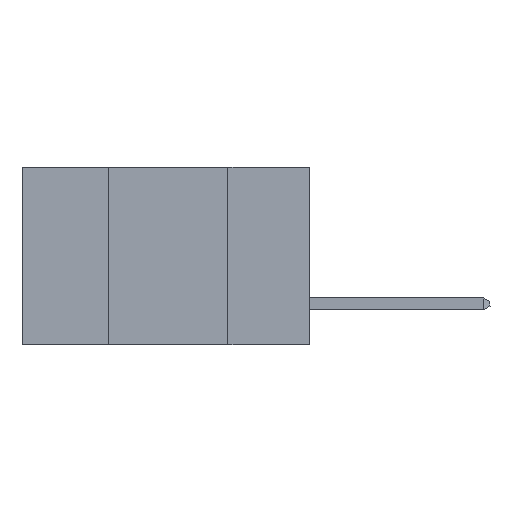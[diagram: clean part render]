
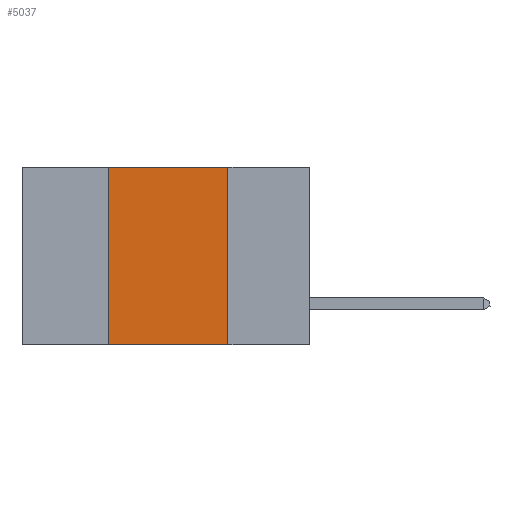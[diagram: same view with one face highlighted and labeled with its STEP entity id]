
A CAD part, left-side view. The second image highlights one B-rep face of the part: STEP entity #5037.
In plain terms, the highlighted planar face has unit normal (-1, 0, 0).
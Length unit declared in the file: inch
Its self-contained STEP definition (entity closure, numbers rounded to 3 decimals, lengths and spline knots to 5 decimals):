
#1005 = VECTOR ( 'NONE', #12761, 39.37008 ) ;
#1248 = FACE_OUTER_BOUND ( 'NONE', #7220, .T. ) ;
#1402 = LINE ( 'NONE', #6856, #10842 ) ;
#1527 = CARTESIAN_POINT ( 'NONE',  ( 0., 0.42, 0. ) ) ;
#2513 = LINE ( 'NONE', #8085, #5678 ) ;
#3950 = CARTESIAN_POINT ( 'NONE',  ( 0., 0.42, -0.37 ) ) ;
#4233 = LINE ( 'NONE', #4594, #1005 ) ;
#4409 = LINE ( 'NONE', #9572, #10308 ) ;
#4428 = VERTEX_POINT ( 'NONE', #9862 ) ;
#4594 = CARTESIAN_POINT ( 'NONE',  ( 0., 0.6, -0.37 ) ) ;
#4673 = AXIS2_PLACEMENT_3D ( 'NONE', #12328, #12309, #12293 ) ;
#4793 = ORIENTED_EDGE ( 'NONE', *, *, #11866, .F. ) ;
#5037 = ADVANCED_FACE ( 'NONE', ( #1248 ), #12649, .F. ) ;
#5542 = ORIENTED_EDGE ( 'NONE', *, *, #11166, .F. ) ;
#5675 = VERTEX_POINT ( 'NONE', #3950 ) ;
#5678 = VECTOR ( 'NONE', #8144, 39.37008 ) ;
#6143 = EDGE_CURVE ( 'NONE', #5675, #4428, #4233, .T. ) ;
#6856 = CARTESIAN_POINT ( 'NONE',  ( 0., 0.6, 0. ) ) ;
#7220 = EDGE_LOOP ( 'NONE', ( #4793, #5542, #12440, #10150 ) ) ;
#8085 = CARTESIAN_POINT ( 'NONE',  ( 0., 0.17, 0. ) ) ;
#8144 = DIRECTION ( 'NONE',  ( 0., 0., -1. ) ) ;
#8832 = VERTEX_POINT ( 'NONE', #1527 ) ;
#9268 = DIRECTION ( 'NONE',  ( 0., -1., 0. ) ) ;
#9572 = CARTESIAN_POINT ( 'NONE',  ( 0., 0.42, 0. ) ) ;
#9862 = CARTESIAN_POINT ( 'NONE',  ( 0., 0.17, -0.37 ) ) ;
#10150 = ORIENTED_EDGE ( 'NONE', *, *, #6143, .T. ) ;
#10308 = VECTOR ( 'NONE', #10802, 39.37008 ) ;
#10802 = DIRECTION ( 'NONE',  ( 0., 0., 1. ) ) ;
#10842 = VECTOR ( 'NONE', #9268, 39.37008 ) ;
#11166 = EDGE_CURVE ( 'NONE', #8832, #13412, #1402, .T. ) ;
#11349 = EDGE_CURVE ( 'NONE', #5675, #8832, #4409, .T. ) ;
#11866 = EDGE_CURVE ( 'NONE', #13412, #4428, #2513, .T. ) ;
#12293 = DIRECTION ( 'NONE',  ( 0., 0., -1. ) ) ;
#12309 = DIRECTION ( 'NONE',  ( 1., 0., 0. ) ) ;
#12328 = CARTESIAN_POINT ( 'NONE',  ( 0., 0.6, 0. ) ) ;
#12395 = CARTESIAN_POINT ( 'NONE',  ( 0., 0.17, 0. ) ) ;
#12440 = ORIENTED_EDGE ( 'NONE', *, *, #11349, .F. ) ;
#12649 = PLANE ( 'NONE',  #4673 ) ;
#12761 = DIRECTION ( 'NONE',  ( 0., -1., 0. ) ) ;
#13412 = VERTEX_POINT ( 'NONE', #12395 ) ;
